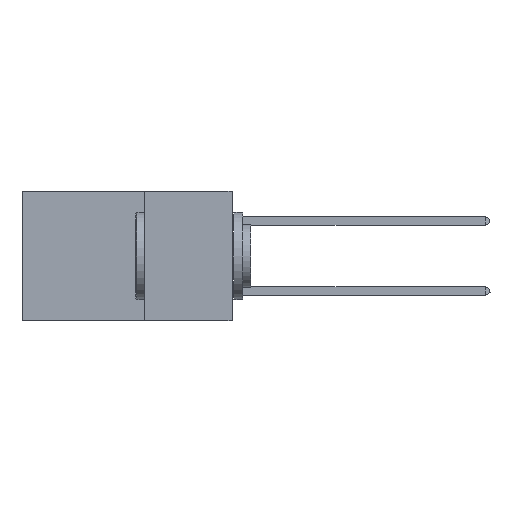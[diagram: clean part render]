
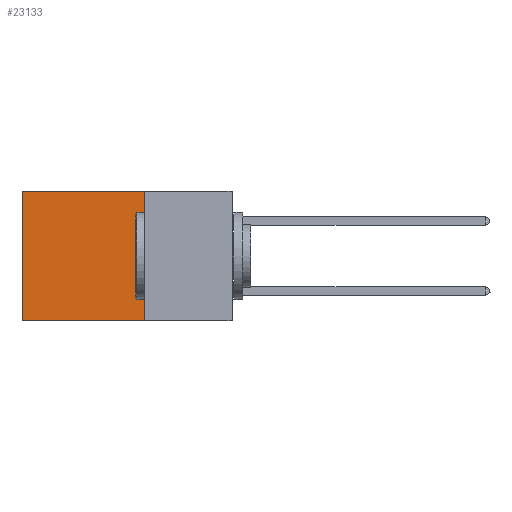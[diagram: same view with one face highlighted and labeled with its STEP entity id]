
A CAD part, left-side view. The second image highlights one B-rep face of the part: STEP entity #23133.
In plain terms, the highlighted planar face has unit normal (-1, 0, 0).
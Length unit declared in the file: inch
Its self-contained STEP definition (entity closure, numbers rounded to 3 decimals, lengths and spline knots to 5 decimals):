
#212 = CARTESIAN_POINT ( 'NONE',  ( 0.2875, 0.25, 0. ) ) ;
#1467 = DIRECTION ( 'NONE',  ( 0., 0., -1. ) ) ;
#1815 = LINE ( 'NONE', #28314, #7555 ) ;
#1894 = VECTOR ( 'NONE', #28937, 39.37008 ) ;
#4039 = VERTEX_POINT ( 'NONE', #212 ) ;
#5847 = EDGE_CURVE ( 'NONE', #29650, #19898, #17673, .T. ) ;
#6201 = EDGE_CURVE ( 'NONE', #37231, #19898, #23406, .T. ) ;
#6825 = ORIENTED_EDGE ( 'NONE', *, *, #6201, .F. ) ;
#7555 = VECTOR ( 'NONE', #42188, 39.37008 ) ;
#8130 = EDGE_CURVE ( 'NONE', #4039, #29650, #14372, .T. ) ;
#10405 = ORIENTED_EDGE ( 'NONE', *, *, #16128, .F. ) ;
#14372 = LINE ( 'NONE', #26010, #1894 ) ;
#15063 = VECTOR ( 'NONE', #41711, 39.37008 ) ;
#15132 = CARTESIAN_POINT ( 'NONE',  ( 0.2875, 0.25, 0. ) ) ;
#16128 = EDGE_CURVE ( 'NONE', #4039, #37231, #1815, .T. ) ;
#16179 = CARTESIAN_POINT ( 'NONE',  ( 0.2875, 0.25, -0.37 ) ) ;
#17673 = LINE ( 'NONE', #24632, #15063 ) ;
#18538 = CARTESIAN_POINT ( 'NONE',  ( 0.2875, 0.6, -0.37 ) ) ;
#19898 = VERTEX_POINT ( 'NONE', #18538 ) ;
#23133 = ADVANCED_FACE ( 'NONE', ( #37996 ), #38066, .F. ) ;
#23297 = EDGE_LOOP ( 'NONE', ( #33634, #6825, #10405, #34028 ) ) ;
#23406 = LINE ( 'NONE', #39368, #28662 ) ;
#24398 = AXIS2_PLACEMENT_3D ( 'NONE', #15132, #38211, #1467 ) ;
#24632 = CARTESIAN_POINT ( 'NONE',  ( 0.2875, 0.6, 0. ) ) ;
#25939 = DIRECTION ( 'NONE',  ( 0., 1., 0. ) ) ;
#26010 = CARTESIAN_POINT ( 'NONE',  ( 0.2875, 0.25, 0. ) ) ;
#28314 = CARTESIAN_POINT ( 'NONE',  ( 0.2875, 0.25, 0. ) ) ;
#28662 = VECTOR ( 'NONE', #25939, 39.37008 ) ;
#28937 = DIRECTION ( 'NONE',  ( 0., 1., 0. ) ) ;
#29650 = VERTEX_POINT ( 'NONE', #36178 ) ;
#33634 = ORIENTED_EDGE ( 'NONE', *, *, #5847, .T. ) ;
#34028 = ORIENTED_EDGE ( 'NONE', *, *, #8130, .T. ) ;
#36178 = CARTESIAN_POINT ( 'NONE',  ( 0.2875, 0.6, 0. ) ) ;
#37231 = VERTEX_POINT ( 'NONE', #16179 ) ;
#37996 = FACE_OUTER_BOUND ( 'NONE', #23297, .T. ) ;
#38066 = PLANE ( 'NONE',  #24398 ) ;
#38211 = DIRECTION ( 'NONE',  ( 1., 0., 0. ) ) ;
#39368 = CARTESIAN_POINT ( 'NONE',  ( 0.2875, 0.25, -0.37 ) ) ;
#41711 = DIRECTION ( 'NONE',  ( 0., 0., -1. ) ) ;
#42188 = DIRECTION ( 'NONE',  ( 0., 0., -1. ) ) ;
